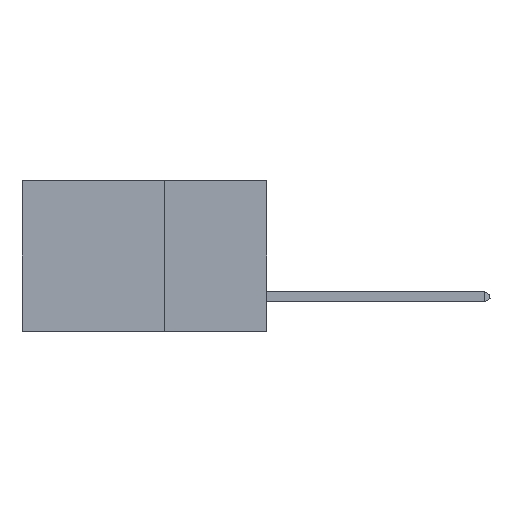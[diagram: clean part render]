
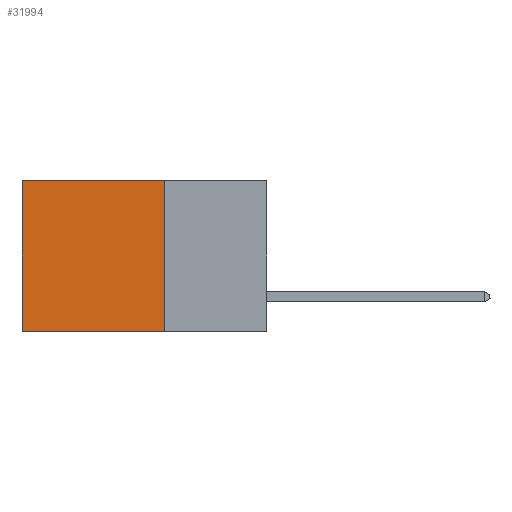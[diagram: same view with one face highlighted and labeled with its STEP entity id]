
A CAD part, left-side view. The second image highlights one B-rep face of the part: STEP entity #31994.
In plain terms, the highlighted planar face has unit normal (-1, 0, 0).
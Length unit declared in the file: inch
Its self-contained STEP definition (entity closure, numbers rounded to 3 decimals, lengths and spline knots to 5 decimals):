
#52 = VERTEX_POINT ( 'NONE', #22589 ) ;
#2333 = ORIENTED_EDGE ( 'NONE', *, *, #26891, .T. ) ;
#2896 = EDGE_CURVE ( 'NONE', #52, #32820, #4146, .T. ) ;
#4146 = LINE ( 'NONE', #32301, #47586 ) ;
#5324 = VECTOR ( 'NONE', #44968, 39.37008 ) ;
#7074 = VERTEX_POINT ( 'NONE', #50052 ) ;
#8859 = FACE_OUTER_BOUND ( 'NONE', #25657, .T. ) ;
#11557 = CARTESIAN_POINT ( 'NONE',  ( 0.2875, 0.6, 0. ) ) ;
#14215 = EDGE_CURVE ( 'NONE', #49667, #7074, #30628, .T. ) ;
#15075 = ORIENTED_EDGE ( 'NONE', *, *, #14215, .T. ) ;
#18836 = PLANE ( 'NONE',  #23540 ) ;
#19341 = DIRECTION ( 'NONE',  ( 1., 0., 0. ) ) ;
#22589 = CARTESIAN_POINT ( 'NONE',  ( 0.2875, 0.25, 0. ) ) ;
#23329 = DIRECTION ( 'NONE',  ( 0., 0., -1. ) ) ;
#23540 = AXIS2_PLACEMENT_3D ( 'NONE', #39088, #19341, #35231 ) ;
#25657 = EDGE_LOOP ( 'NONE', ( #15075, #34568, #47786, #2333 ) ) ;
#26891 = EDGE_CURVE ( 'NONE', #52, #49667, #32153, .T. ) ;
#29674 = VECTOR ( 'NONE', #34135, 39.37008 ) ;
#30628 = LINE ( 'NONE', #11557, #43692 ) ;
#31994 = ADVANCED_FACE ( 'NONE', ( #8859 ), #18836, .F. ) ;
#32153 = LINE ( 'NONE', #42144, #29674 ) ;
#32301 = CARTESIAN_POINT ( 'NONE',  ( 0.2875, 0.25, 0. ) ) ;
#32820 = VERTEX_POINT ( 'NONE', #43857 ) ;
#34135 = DIRECTION ( 'NONE',  ( 0., 1., 0. ) ) ;
#34472 = LINE ( 'NONE', #37337, #5324 ) ;
#34568 = ORIENTED_EDGE ( 'NONE', *, *, #45995, .F. ) ;
#35231 = DIRECTION ( 'NONE',  ( 0., 0., -1. ) ) ;
#36640 = DIRECTION ( 'NONE',  ( 0., 0., -1. ) ) ;
#37337 = CARTESIAN_POINT ( 'NONE',  ( 0.2875, 0.25, -0.37 ) ) ;
#39088 = CARTESIAN_POINT ( 'NONE',  ( 0.2875, 0.25, 0. ) ) ;
#42144 = CARTESIAN_POINT ( 'NONE',  ( 0.2875, 0.25, 0. ) ) ;
#43692 = VECTOR ( 'NONE', #23329, 39.37008 ) ;
#43857 = CARTESIAN_POINT ( 'NONE',  ( 0.2875, 0.25, -0.37 ) ) ;
#44968 = DIRECTION ( 'NONE',  ( 0., 1., 0. ) ) ;
#45995 = EDGE_CURVE ( 'NONE', #32820, #7074, #34472, .T. ) ;
#47586 = VECTOR ( 'NONE', #36640, 39.37008 ) ;
#47786 = ORIENTED_EDGE ( 'NONE', *, *, #2896, .F. ) ;
#48408 = CARTESIAN_POINT ( 'NONE',  ( 0.2875, 0.6, 0. ) ) ;
#49667 = VERTEX_POINT ( 'NONE', #48408 ) ;
#50052 = CARTESIAN_POINT ( 'NONE',  ( 0.2875, 0.6, -0.37 ) ) ;
